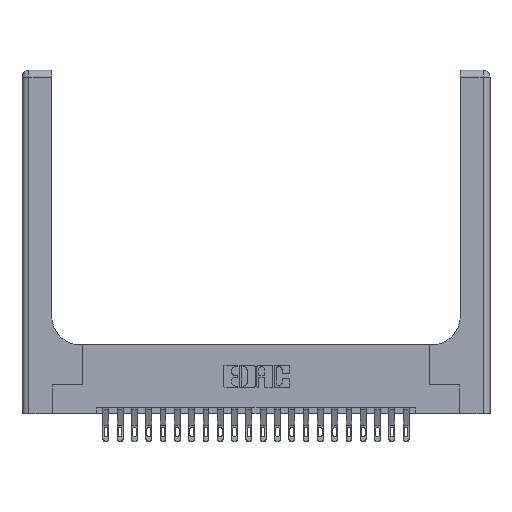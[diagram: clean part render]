
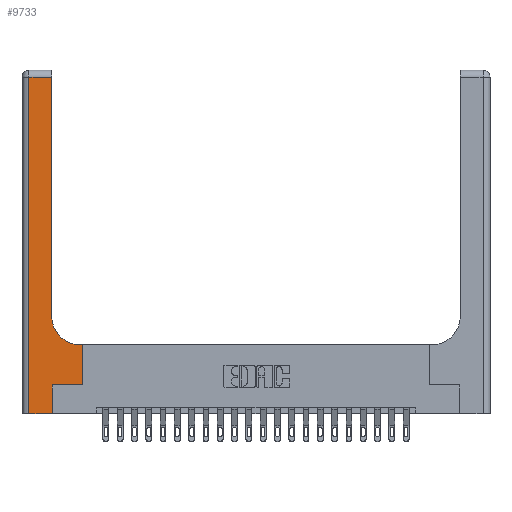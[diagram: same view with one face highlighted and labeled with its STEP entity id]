
A CAD part, top view. The second image highlights one B-rep face of the part: STEP entity #9733.
In plain terms, the highlighted planar face has unit normal (0, 0, 1).
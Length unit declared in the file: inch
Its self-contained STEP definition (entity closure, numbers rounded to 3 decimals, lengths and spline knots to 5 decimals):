
#897 = CARTESIAN_POINT ( 'NONE',  ( 0.26, 0.85, 0.37 ) ) ;
#1050 = VERTEX_POINT ( 'NONE', #4827 ) ;
#1090 = ORIENTED_EDGE ( 'NONE', *, *, #7407, .T. ) ;
#1858 = CARTESIAN_POINT ( 'NONE',  ( 0.528, 0.6, 0.37 ) ) ;
#2302 = PLANE ( 'NONE',  #3533 ) ;
#2330 = VECTOR ( 'NONE', #21431, 39.37008 ) ;
#2425 = CARTESIAN_POINT ( 'NONE',  ( 0., 3., 0.37 ) ) ;
#3066 = LINE ( 'NONE', #15411, #9240 ) ;
#3317 = CARTESIAN_POINT ( 'NONE',  ( 0.51, 0.6, 0.37 ) ) ;
#3517 = VECTOR ( 'NONE', #11636, 39.37008 ) ;
#3533 = AXIS2_PLACEMENT_3D ( 'NONE', #2425, #16516, #9570 ) ;
#3572 = CARTESIAN_POINT ( 'NONE',  ( 0., 2.94, 0.37 ) ) ;
#4006 = VECTOR ( 'NONE', #14333, 39.37008 ) ;
#4827 = CARTESIAN_POINT ( 'NONE',  ( 0.265, 0.25, 0.37 ) ) ;
#5190 = ORIENTED_EDGE ( 'NONE', *, *, #8762, .T. ) ;
#5288 = VERTEX_POINT ( 'NONE', #12294 ) ;
#5681 = EDGE_CURVE ( 'NONE', #5288, #12108, #9348, .T. ) ;
#5806 = EDGE_CURVE ( 'NONE', #17561, #9227, #18519, .T. ) ;
#5950 = EDGE_CURVE ( 'NONE', #11596, #22843, #21381, .T. ) ;
#5983 = EDGE_LOOP ( 'NONE', ( #8294, #21338, #1090, #7753, #5190, #16280, #9746, #13350, #20291 ) ) ;
#6393 = EDGE_CURVE ( 'NONE', #9227, #19471, #22439, .T. ) ;
#6493 = DIRECTION ( 'NONE',  ( 0., 1., 0. ) ) ;
#6641 = DIRECTION ( 'NONE',  ( 0., 1., 0. ) ) ;
#7072 = DIRECTION ( 'NONE',  ( 1., 0., 0. ) ) ;
#7249 = CARTESIAN_POINT ( 'NONE',  ( 0.265, 0.25, 0.37 ) ) ;
#7407 = EDGE_CURVE ( 'NONE', #22843, #5288, #13042, .T. ) ;
#7753 = ORIENTED_EDGE ( 'NONE', *, *, #5681, .T. ) ;
#8052 = CARTESIAN_POINT ( 'NONE',  ( 0.26, 2.94, 0.37 ) ) ;
#8294 = ORIENTED_EDGE ( 'NONE', *, *, #18118, .T. ) ;
#8762 = EDGE_CURVE ( 'NONE', #12108, #1050, #13845, .T. ) ;
#9124 = CARTESIAN_POINT ( 'NONE',  ( 0.528, 0.25, 0.37 ) ) ;
#9227 = VERTEX_POINT ( 'NONE', #3317 ) ;
#9239 = CARTESIAN_POINT ( 'NONE',  ( 0.06, 2.94, 0.37 ) ) ;
#9240 = VECTOR ( 'NONE', #6493, 39.37008 ) ;
#9348 = LINE ( 'NONE', #10748, #2330 ) ;
#9570 = DIRECTION ( 'NONE',  ( -1., 0., 0. ) ) ;
#9699 = DIRECTION ( 'NONE',  ( -1., 0., 0. ) ) ;
#9733 = ADVANCED_FACE ( 'NONE', ( #13046 ), #2302, .F. ) ;
#9746 = ORIENTED_EDGE ( 'NONE', *, *, #15816, .T. ) ;
#9904 = CARTESIAN_POINT ( 'NONE',  ( 0.06, 3., 0.37 ) ) ;
#10571 = AXIS2_PLACEMENT_3D ( 'NONE', #15865, #22967, #7072 ) ;
#10583 = DIRECTION ( 'NONE',  ( -1., 0., 0. ) ) ;
#10748 = CARTESIAN_POINT ( 'NONE',  ( 0., 0., 0.37 ) ) ;
#10808 = LINE ( 'NONE', #12664, #13021 ) ;
#10923 = DIRECTION ( 'NONE',  ( 0., 1., 0. ) ) ;
#11596 = VERTEX_POINT ( 'NONE', #8052 ) ;
#11636 = DIRECTION ( 'NONE',  ( 0., -1., 0. ) ) ;
#11984 = CARTESIAN_POINT ( 'NONE',  ( 0.265, 0., 0.37 ) ) ;
#12108 = VERTEX_POINT ( 'NONE', #20491 ) ;
#12294 = CARTESIAN_POINT ( 'NONE',  ( 0.06, 0., 0.37 ) ) ;
#12664 = CARTESIAN_POINT ( 'NONE',  ( 0.26, 3., 0.37 ) ) ;
#12997 = VECTOR ( 'NONE', #10583, 39.37008 ) ;
#13021 = VECTOR ( 'NONE', #10923, 39.37008 ) ;
#13042 = LINE ( 'NONE', #9904, #3517 ) ;
#13046 = FACE_OUTER_BOUND ( 'NONE', #5983, .T. ) ;
#13350 = ORIENTED_EDGE ( 'NONE', *, *, #5806, .T. ) ;
#13452 = EDGE_CURVE ( 'NONE', #1050, #22834, #15936, .T. ) ;
#13562 = VECTOR ( 'NONE', #6641, 39.37008 ) ;
#13845 = LINE ( 'NONE', #11984, #13562 ) ;
#14333 = DIRECTION ( 'NONE',  ( 1., 0., 0. ) ) ;
#15411 = CARTESIAN_POINT ( 'NONE',  ( 0.528, 0.25, 0.37 ) ) ;
#15816 = EDGE_CURVE ( 'NONE', #22834, #17561, #3066, .T. ) ;
#15865 = CARTESIAN_POINT ( 'NONE',  ( 0.51, 0.85, 0.37 ) ) ;
#15936 = LINE ( 'NONE', #7249, #4006 ) ;
#16280 = ORIENTED_EDGE ( 'NONE', *, *, #13452, .T. ) ;
#16516 = DIRECTION ( 'NONE',  ( 0., 0., -1. ) ) ;
#17561 = VERTEX_POINT ( 'NONE', #1858 ) ;
#18118 = EDGE_CURVE ( 'NONE', #19471, #11596, #10808, .T. ) ;
#18407 = CARTESIAN_POINT ( 'NONE',  ( 0.26, 0.6, 0.37 ) ) ;
#18519 = LINE ( 'NONE', #18407, #22815 ) ;
#19471 = VERTEX_POINT ( 'NONE', #897 ) ;
#20291 = ORIENTED_EDGE ( 'NONE', *, *, #6393, .T. ) ;
#20491 = CARTESIAN_POINT ( 'NONE',  ( 0.265, 0., 0.37 ) ) ;
#21338 = ORIENTED_EDGE ( 'NONE', *, *, #5950, .T. ) ;
#21381 = LINE ( 'NONE', #3572, #12997 ) ;
#21431 = DIRECTION ( 'NONE',  ( 1., 0., 0. ) ) ;
#22439 = CIRCLE ( 'NONE', #10571, 0.25 ) ;
#22815 = VECTOR ( 'NONE', #9699, 39.37008 ) ;
#22834 = VERTEX_POINT ( 'NONE', #9124 ) ;
#22843 = VERTEX_POINT ( 'NONE', #9239 ) ;
#22967 = DIRECTION ( 'NONE',  ( 0., 0., -1. ) ) ;
